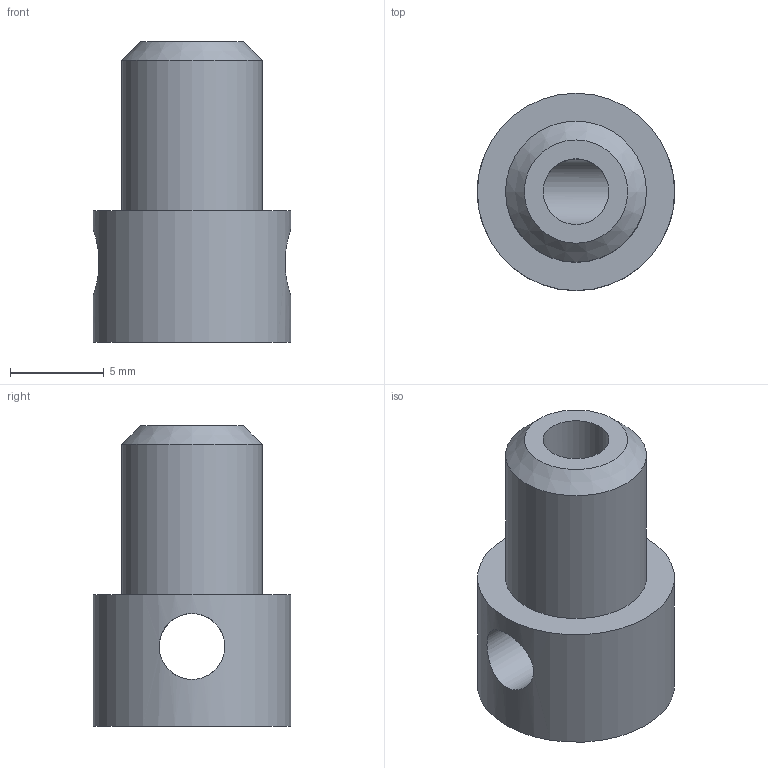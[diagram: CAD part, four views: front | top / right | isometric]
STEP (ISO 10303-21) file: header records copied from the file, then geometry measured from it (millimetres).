
FILE_DESCRIPTION( ( '' ), ' ' );
FILE_NAME( '5dc6e35094333712756289d2.step', '2019-11-09T16:03:28', ( '' ), ( '' ), ' ', ' ', ' ' );
FILE_SCHEMA( ( 'AUTOMOTIVE_DESIGN { 1 0 10303 214 1 1 1 1 }' ) );
Length unit declared in the file: metre
Products named in the file (1): Part 1
Bounding box: 10.5 x 10.5 x 16 mm (x, y, z)
Volume: 757.1 mm3; surface area: 824.1 mm2
Topology: 1 solids, 1 shells, 12 faces, 24 edges, 16 vertices
Faces by surface type: cylinder 6, plane 5, cone 1
Full cylindrical faces by diameter (mm): 3.5 x3, 7.5 x1, 7.75 x1, 10.5 x1
Entity records: 488 total; most frequent: CARTESIAN_POINT 151, DIRECTION 50, ORIENTED_EDGE 28, EDGE_LOOP 26, AXIS2_PLACEMENT_3D 25, FACE_OUTER_BOUND 18, EDGE_CURVE 14, VERTEX_POINT 14
